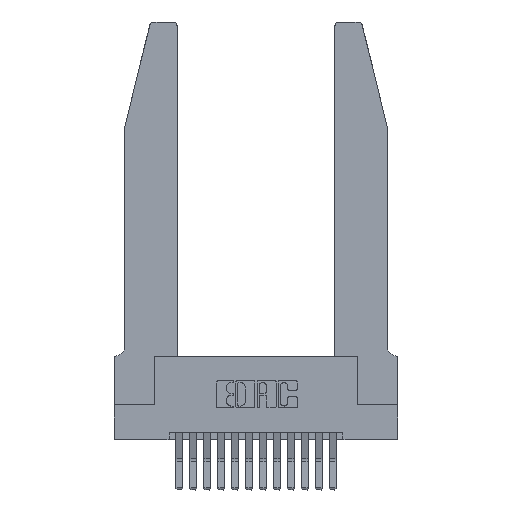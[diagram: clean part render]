
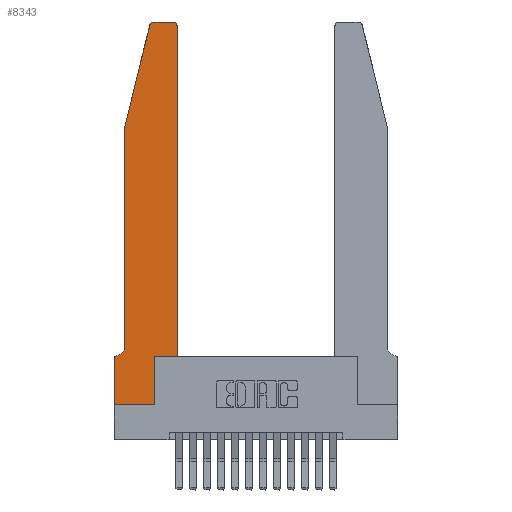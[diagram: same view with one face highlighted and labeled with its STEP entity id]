
A CAD part, top view. The second image highlights one B-rep face of the part: STEP entity #8343.
In plain terms, the highlighted planar face has unit normal (0, 0, 1).
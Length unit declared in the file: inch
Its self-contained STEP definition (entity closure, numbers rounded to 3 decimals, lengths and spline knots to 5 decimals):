
#30 = ORIENTED_EDGE ( 'NONE', *, *, #5017, .T. ) ;
#138 = CARTESIAN_POINT ( 'NONE',  ( 0.0755, 2., 0.37 ) ) ;
#367 = CARTESIAN_POINT ( 'NONE',  ( 0., 0., 0.37 ) ) ;
#428 = ORIENTED_EDGE ( 'NONE', *, *, #14783, .T. ) ;
#507 = LINE ( 'NONE', #14464, #2246 ) ;
#628 = EDGE_CURVE ( 'NONE', #12281, #1635, #9262, .T. ) ;
#705 = ORIENTED_EDGE ( 'NONE', *, *, #6768, .T. ) ;
#829 = CARTESIAN_POINT ( 'NONE',  ( 0.4505, 2.72, 0.37 ) ) ;
#1465 = CARTESIAN_POINT ( 'NONE',  ( 0.0755, 0.35, 0.37 ) ) ;
#1635 = VERTEX_POINT ( 'NONE', #7638 ) ;
#1941 = CARTESIAN_POINT ( 'NONE',  ( 0.2865, 0.35, 0.37 ) ) ;
#1989 = AXIS2_PLACEMENT_3D ( 'NONE', #4671, #4787, #2014 ) ;
#2014 = DIRECTION ( 'NONE',  ( -1., 0., 0. ) ) ;
#2016 = EDGE_CURVE ( 'NONE', #5320, #14356, #12534, .T. ) ;
#2088 = CARTESIAN_POINT ( 'NONE',  ( 0.2865, 0.35, 0.37 ) ) ;
#2218 = EDGE_CURVE ( 'NONE', #11944, #5320, #10344, .T. ) ;
#2246 = VECTOR ( 'NONE', #3424, 39.37008 ) ;
#2451 = PLANE ( 'NONE',  #10554 ) ;
#2552 = DIRECTION ( 'NONE',  ( 1., 0., 0. ) ) ;
#2642 = LINE ( 'NONE', #1465, #11946 ) ;
#3059 = ORIENTED_EDGE ( 'NONE', *, *, #13036, .T. ) ;
#3119 = LINE ( 'NONE', #18134, #12832 ) ;
#3231 = LINE ( 'NONE', #367, #14025 ) ;
#3270 = VERTEX_POINT ( 'NONE', #16170 ) ;
#3419 = ORIENTED_EDGE ( 'NONE', *, *, #2016, .T. ) ;
#3424 = DIRECTION ( 'NONE',  ( 0., -1., 0. ) ) ;
#4230 = VERTEX_POINT ( 'NONE', #11351 ) ;
#4671 = CARTESIAN_POINT ( 'NONE',  ( 0.0055, 0.42, 0.37 ) ) ;
#4708 = LINE ( 'NONE', #17590, #11995 ) ;
#4787 = DIRECTION ( 'NONE',  ( 0., 0., -1. ) ) ;
#5017 = EDGE_CURVE ( 'NONE', #4230, #16864, #3231, .T. ) ;
#5158 = EDGE_LOOP ( 'NONE', ( #6347, #12865, #18019, #3419, #428, #9305, #705, #30, #12386, #3059, #12192, #8782 ) ) ;
#5317 = VECTOR ( 'NONE', #17471, 39.37008 ) ;
#5320 = VERTEX_POINT ( 'NONE', #17023 ) ;
#5436 = DIRECTION ( 'NONE',  ( 0., -1., 0. ) ) ;
#5481 = AXIS2_PLACEMENT_3D ( 'NONE', #12368, #13788, #9419 ) ;
#5492 = CARTESIAN_POINT ( 'NONE',  ( 0.4205, 2.75, 0.37 ) ) ;
#6093 = VERTEX_POINT ( 'NONE', #829 ) ;
#6347 = ORIENTED_EDGE ( 'NONE', *, *, #628, .T. ) ;
#6553 = DIRECTION ( 'NONE',  ( 1., 0., 0. ) ) ;
#6768 = EDGE_CURVE ( 'NONE', #11427, #4230, #507, .T. ) ;
#6967 = CARTESIAN_POINT ( 'NONE',  ( 0.0755, 2., 0.37 ) ) ;
#7484 = CARTESIAN_POINT ( 'NONE',  ( 0.25487, 2.72718, 0.37 ) ) ;
#7638 = CARTESIAN_POINT ( 'NONE',  ( 0.284, 2.75, 0.37 ) ) ;
#8343 = ADVANCED_FACE ( 'NONE', ( #12131 ), #2451, .T. ) ;
#8782 = ORIENTED_EDGE ( 'NONE', *, *, #15534, .T. ) ;
#9256 = CARTESIAN_POINT ( 'NONE',  ( 0.0755, 0.42, 0.37 ) ) ;
#9262 = LINE ( 'NONE', #12320, #16340 ) ;
#9305 = ORIENTED_EDGE ( 'NONE', *, *, #18055, .T. ) ;
#9419 = DIRECTION ( 'NONE',  ( 1., 0., 0. ) ) ;
#9460 = AXIS2_PLACEMENT_3D ( 'NONE', #13653, #12423, #2552 ) ;
#9920 = DIRECTION ( 'NONE',  ( -1., 0., 0. ) ) ;
#10051 = CARTESIAN_POINT ( 'NONE',  ( 0.2865, 0., 0.37 ) ) ;
#10344 = LINE ( 'NONE', #138, #15189 ) ;
#10511 = CARTESIAN_POINT ( 'NONE',  ( 0.0055, 0.35, 0.37 ) ) ;
#10554 = AXIS2_PLACEMENT_3D ( 'NONE', #13559, #17920, #16418 ) ;
#11098 = DIRECTION ( 'NONE',  ( -1., 0., 0. ) ) ;
#11351 = CARTESIAN_POINT ( 'NONE',  ( 0., 0., 0.37 ) ) ;
#11427 = VERTEX_POINT ( 'NONE', #15854 ) ;
#11753 = EDGE_CURVE ( 'NONE', #1635, #11944, #16664, .T. ) ;
#11896 = VECTOR ( 'NONE', #5436, 39.37008 ) ;
#11944 = VERTEX_POINT ( 'NONE', #7484 ) ;
#11946 = VECTOR ( 'NONE', #11098, 39.37008 ) ;
#11995 = VECTOR ( 'NONE', #13406, 39.37008 ) ;
#11996 = EDGE_CURVE ( 'NONE', #3270, #6093, #4708, .T. ) ;
#12131 = FACE_OUTER_BOUND ( 'NONE', #5158, .T. ) ;
#12192 = ORIENTED_EDGE ( 'NONE', *, *, #11996, .T. ) ;
#12281 = VERTEX_POINT ( 'NONE', #5492 ) ;
#12320 = CARTESIAN_POINT ( 'NONE',  ( 0.2605, 2.75, 0.37 ) ) ;
#12368 = CARTESIAN_POINT ( 'NONE',  ( 0.284, 2.72, 0.37 ) ) ;
#12386 = ORIENTED_EDGE ( 'NONE', *, *, #17071, .T. ) ;
#12423 = DIRECTION ( 'NONE',  ( 0., 0., 1. ) ) ;
#12534 = LINE ( 'NONE', #6967, #11896 ) ;
#12832 = VECTOR ( 'NONE', #6553, 39.37008 ) ;
#12865 = ORIENTED_EDGE ( 'NONE', *, *, #11753, .T. ) ;
#13036 = EDGE_CURVE ( 'NONE', #16492, #3270, #3119, .T. ) ;
#13406 = DIRECTION ( 'NONE',  ( 0., 1., 0. ) ) ;
#13559 = CARTESIAN_POINT ( 'NONE',  ( 0., 0.35, 0.37 ) ) ;
#13653 = CARTESIAN_POINT ( 'NONE',  ( 0.4205, 2.72, 0.37 ) ) ;
#13788 = DIRECTION ( 'NONE',  ( 0., 0., 1. ) ) ;
#13843 = CIRCLE ( 'NONE', #9460, 0.03 ) ;
#14025 = VECTOR ( 'NONE', #14496, 39.37008 ) ;
#14208 = DIRECTION ( 'NONE',  ( -0.239, -0.971, 0. ) ) ;
#14356 = VERTEX_POINT ( 'NONE', #9256 ) ;
#14464 = CARTESIAN_POINT ( 'NONE',  ( 0., 0., 0.37 ) ) ;
#14496 = DIRECTION ( 'NONE',  ( 1., 0., 0. ) ) ;
#14783 = EDGE_CURVE ( 'NONE', #14356, #15932, #16090, .T. ) ;
#15189 = VECTOR ( 'NONE', #14208, 39.37008 ) ;
#15534 = EDGE_CURVE ( 'NONE', #6093, #12281, #13843, .T. ) ;
#15854 = CARTESIAN_POINT ( 'NONE',  ( 0., 0.35, 0.37 ) ) ;
#15932 = VERTEX_POINT ( 'NONE', #10511 ) ;
#16090 = CIRCLE ( 'NONE', #1989, 0.07 ) ;
#16170 = CARTESIAN_POINT ( 'NONE',  ( 0.4505, 0.35, 0.37 ) ) ;
#16340 = VECTOR ( 'NONE', #9920, 39.37008 ) ;
#16418 = DIRECTION ( 'NONE',  ( 1., 0., 0. ) ) ;
#16492 = VERTEX_POINT ( 'NONE', #2088 ) ;
#16664 = CIRCLE ( 'NONE', #5481, 0.03 ) ;
#16864 = VERTEX_POINT ( 'NONE', #10051 ) ;
#17023 = CARTESIAN_POINT ( 'NONE',  ( 0.0755, 2., 0.37 ) ) ;
#17071 = EDGE_CURVE ( 'NONE', #16864, #16492, #17956, .T. ) ;
#17471 = DIRECTION ( 'NONE',  ( 0., 1., 0. ) ) ;
#17590 = CARTESIAN_POINT ( 'NONE',  ( 0.4505, 0.35, 0.37 ) ) ;
#17920 = DIRECTION ( 'NONE',  ( 0., 0., 1. ) ) ;
#17956 = LINE ( 'NONE', #1941, #5317 ) ;
#18019 = ORIENTED_EDGE ( 'NONE', *, *, #2218, .T. ) ;
#18055 = EDGE_CURVE ( 'NONE', #15932, #11427, #2642, .T. ) ;
#18134 = CARTESIAN_POINT ( 'NONE',  ( 0.4505, 0.35, 0.37 ) ) ;
